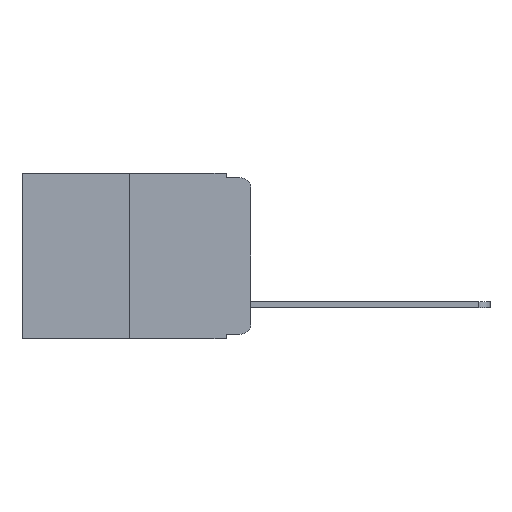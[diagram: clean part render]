
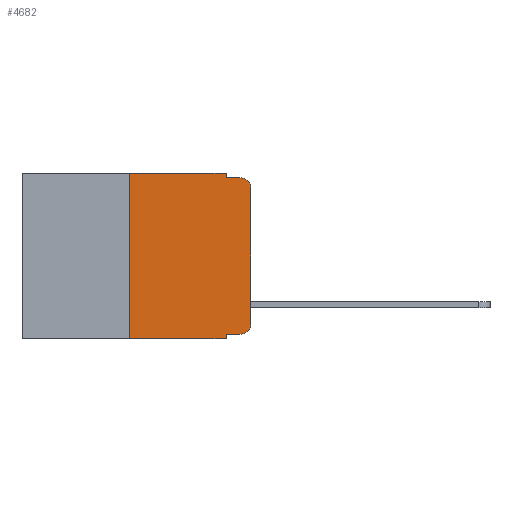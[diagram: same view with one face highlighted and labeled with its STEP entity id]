
A CAD part, left-side view. The second image highlights one B-rep face of the part: STEP entity #4682.
In plain terms, the highlighted planar face has unit normal (-1, 0, 0).
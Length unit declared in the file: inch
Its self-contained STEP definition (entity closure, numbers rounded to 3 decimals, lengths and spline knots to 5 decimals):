
#284 = CARTESIAN_POINT ( 'NONE',  ( 0., 0., 0. ) ) ;
#320 = CIRCLE ( 'NONE', #14981, 0.02 ) ;
#657 = CARTESIAN_POINT ( 'NONE',  ( 0., 0., -0.03 ) ) ;
#1395 = EDGE_CURVE ( 'NONE', #11980, #3252, #5874, .T. ) ;
#1489 = DIRECTION ( 'NONE',  ( -1., 0., 0. ) ) ;
#1631 = ORIENTED_EDGE ( 'NONE', *, *, #5943, .F. ) ;
#2164 = DIRECTION ( 'NONE',  ( 1., 0., 0. ) ) ;
#2286 = VERTEX_POINT ( 'NONE', #15735 ) ;
#2400 = VECTOR ( 'NONE', #16446, 39.37008 ) ;
#3023 = DIRECTION ( 'NONE',  ( 0., 0., 1. ) ) ;
#3252 = VERTEX_POINT ( 'NONE', #4410 ) ;
#3597 = CARTESIAN_POINT ( 'NONE',  ( 0., 0.051, -0.01 ) ) ;
#3799 = EDGE_CURVE ( 'NONE', #10144, #4645, #9888, .T. ) ;
#3830 = EDGE_CURVE ( 'NONE', #10354, #13346, #13795, .T. ) ;
#4078 = LINE ( 'NONE', #284, #5535 ) ;
#4321 = ORIENTED_EDGE ( 'NONE', *, *, #15706, .T. ) ;
#4410 = CARTESIAN_POINT ( 'NONE',  ( 0., 0.02, -0.01 ) ) ;
#4589 = EDGE_CURVE ( 'NONE', #4645, #11980, #8854, .T. ) ;
#4594 = CARTESIAN_POINT ( 'NONE',  ( 0., 0.02, -0.313 ) ) ;
#4645 = VERTEX_POINT ( 'NONE', #8624 ) ;
#4682 = ADVANCED_FACE ( 'NONE', ( #6044 ), #12686, .F. ) ;
#4766 = ORIENTED_EDGE ( 'NONE', *, *, #12106, .T. ) ;
#4788 = LINE ( 'NONE', #11944, #16403 ) ;
#4832 = EDGE_CURVE ( 'NONE', #12584, #13346, #14373, .T. ) ;
#5430 = VECTOR ( 'NONE', #9795, 39.37008 ) ;
#5445 = AXIS2_PLACEMENT_3D ( 'NONE', #16584, #2164, #11294 ) ;
#5535 = VECTOR ( 'NONE', #3023, 39.37008 ) ;
#5612 = CARTESIAN_POINT ( 'NONE',  ( 0., 0.25, 0. ) ) ;
#5626 = VECTOR ( 'NONE', #14275, 39.37008 ) ;
#5778 = AXIS2_PLACEMENT_3D ( 'NONE', #4594, #14920, #7090 ) ;
#5874 = LINE ( 'NONE', #3597, #7254 ) ;
#5916 = ORIENTED_EDGE ( 'NONE', *, *, #8577, .T. ) ;
#5943 = EDGE_CURVE ( 'NONE', #12584, #10144, #12918, .T. ) ;
#5962 = EDGE_CURVE ( 'NONE', #10354, #14514, #4788, .T. ) ;
#6044 = FACE_OUTER_BOUND ( 'NONE', #10807, .T. ) ;
#7090 = DIRECTION ( 'NONE',  ( 0., 0., -1. ) ) ;
#7254 = VECTOR ( 'NONE', #10102, 39.37008 ) ;
#7462 = VERTEX_POINT ( 'NONE', #657 ) ;
#7709 = ORIENTED_EDGE ( 'NONE', *, *, #1395, .F. ) ;
#8201 = DIRECTION ( 'NONE',  ( 0., -1., 0. ) ) ;
#8233 = VECTOR ( 'NONE', #9320, 39.37008 ) ;
#8488 = VECTOR ( 'NONE', #15010, 39.37008 ) ;
#8577 = EDGE_CURVE ( 'NONE', #2286, #7462, #4078, .T. ) ;
#8624 = CARTESIAN_POINT ( 'NONE',  ( 0., 0.051, 0. ) ) ;
#8854 = LINE ( 'NONE', #16359, #5430 ) ;
#9189 = ORIENTED_EDGE ( 'NONE', *, *, #5962, .T. ) ;
#9320 = DIRECTION ( 'NONE',  ( 0., 0., 1. ) ) ;
#9795 = DIRECTION ( 'NONE',  ( 0., 0., -1. ) ) ;
#9885 = CARTESIAN_POINT ( 'NONE',  ( 0., 0.051, -0.343 ) ) ;
#9888 = LINE ( 'NONE', #12195, #8488 ) ;
#10102 = DIRECTION ( 'NONE',  ( 0., -1., 0. ) ) ;
#10144 = VERTEX_POINT ( 'NONE', #14352 ) ;
#10199 = CARTESIAN_POINT ( 'NONE',  ( 0., 0.473, -0.343 ) ) ;
#10354 = VERTEX_POINT ( 'NONE', #11783 ) ;
#10492 = ORIENTED_EDGE ( 'NONE', *, *, #4832, .T. ) ;
#10807 = EDGE_LOOP ( 'NONE', ( #5916, #4321, #7709, #14437, #12869, #1631, #10492, #13520, #9189, #4766 ) ) ;
#11294 = DIRECTION ( 'NONE',  ( 0., 0., -1. ) ) ;
#11767 = CARTESIAN_POINT ( 'NONE',  ( 0., 0.02, -0.03 ) ) ;
#11783 = CARTESIAN_POINT ( 'NONE',  ( 0., 0.051, -0.333 ) ) ;
#11944 = CARTESIAN_POINT ( 'NONE',  ( 0., 0.051, -0.333 ) ) ;
#11980 = VERTEX_POINT ( 'NONE', #15978 ) ;
#12044 = CARTESIAN_POINT ( 'NONE',  ( 0., 0.051, 0. ) ) ;
#12106 = EDGE_CURVE ( 'NONE', #14514, #2286, #14572, .T. ) ;
#12195 = CARTESIAN_POINT ( 'NONE',  ( 0., 0.473, 0. ) ) ;
#12584 = VERTEX_POINT ( 'NONE', #16235 ) ;
#12686 = PLANE ( 'NONE',  #5445 ) ;
#12869 = ORIENTED_EDGE ( 'NONE', *, *, #3799, .F. ) ;
#12918 = LINE ( 'NONE', #5612, #8233 ) ;
#13170 = CARTESIAN_POINT ( 'NONE',  ( 0., 0.02, -0.333 ) ) ;
#13346 = VERTEX_POINT ( 'NONE', #9885 ) ;
#13520 = ORIENTED_EDGE ( 'NONE', *, *, #3830, .F. ) ;
#13795 = LINE ( 'NONE', #12044, #2400 ) ;
#14275 = DIRECTION ( 'NONE',  ( 0., -1., 0. ) ) ;
#14352 = CARTESIAN_POINT ( 'NONE',  ( 0., 0.25, 0. ) ) ;
#14373 = LINE ( 'NONE', #10199, #5626 ) ;
#14437 = ORIENTED_EDGE ( 'NONE', *, *, #4589, .F. ) ;
#14514 = VERTEX_POINT ( 'NONE', #13170 ) ;
#14572 = CIRCLE ( 'NONE', #5778, 0.02 ) ;
#14920 = DIRECTION ( 'NONE',  ( -1., 0., 0. ) ) ;
#14981 = AXIS2_PLACEMENT_3D ( 'NONE', #11767, #1489, #15759 ) ;
#15010 = DIRECTION ( 'NONE',  ( 0., -1., 0. ) ) ;
#15706 = EDGE_CURVE ( 'NONE', #7462, #3252, #320, .T. ) ;
#15735 = CARTESIAN_POINT ( 'NONE',  ( 0., 0., -0.313 ) ) ;
#15759 = DIRECTION ( 'NONE',  ( 0., 0., -1. ) ) ;
#15978 = CARTESIAN_POINT ( 'NONE',  ( 0., 0.051, -0.01 ) ) ;
#16235 = CARTESIAN_POINT ( 'NONE',  ( 0., 0.25, -0.343 ) ) ;
#16359 = CARTESIAN_POINT ( 'NONE',  ( 0., 0.051, 0. ) ) ;
#16403 = VECTOR ( 'NONE', #8201, 39.37008 ) ;
#16446 = DIRECTION ( 'NONE',  ( 0., 0., -1. ) ) ;
#16584 = CARTESIAN_POINT ( 'NONE',  ( 0., 0.473, 0. ) ) ;
